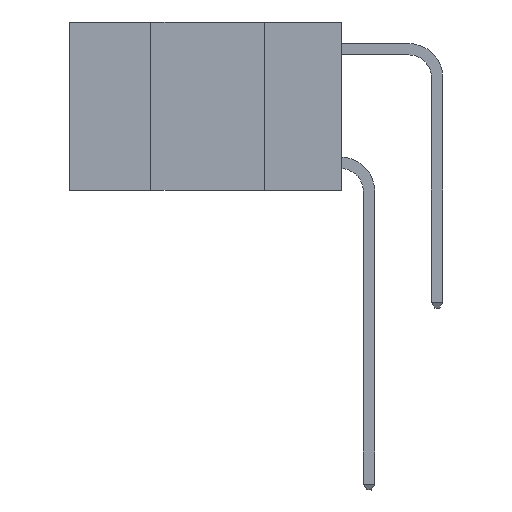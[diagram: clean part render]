
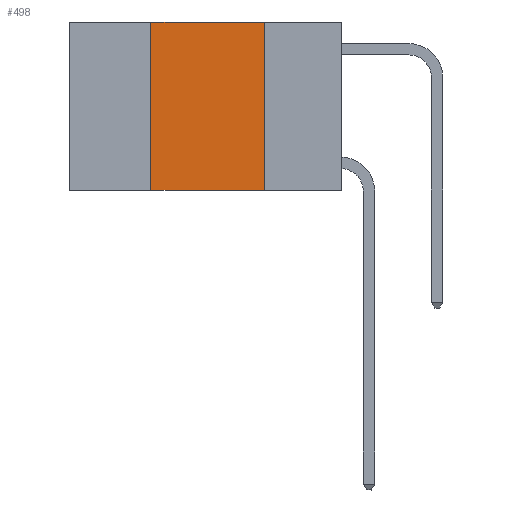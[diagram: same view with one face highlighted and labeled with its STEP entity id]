
A CAD part, left-side view. The second image highlights one B-rep face of the part: STEP entity #498.
In plain terms, the highlighted planar face has unit normal (-1, 0, 0).
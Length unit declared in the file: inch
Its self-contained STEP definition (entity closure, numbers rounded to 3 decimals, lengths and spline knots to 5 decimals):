
#15 = FACE_OUTER_BOUND ( 'NONE', #18554, .T. ) ;
#402 = DIRECTION ( 'NONE',  ( 0., -1., 0. ) ) ;
#498 = ADVANCED_FACE ( 'NONE', ( #15 ), #17483, .F. ) ;
#535 = DIRECTION ( 'NONE',  ( 0., 0., -1. ) ) ;
#1067 = VERTEX_POINT ( 'NONE', #10065 ) ;
#1711 = CARTESIAN_POINT ( 'NONE',  ( 0., 0.17, -0.37 ) ) ;
#2541 = VERTEX_POINT ( 'NONE', #13955 ) ;
#2792 = VERTEX_POINT ( 'NONE', #15150 ) ;
#3217 = LINE ( 'NONE', #16419, #7668 ) ;
#3289 = LINE ( 'NONE', #13831, #11334 ) ;
#4571 = ORIENTED_EDGE ( 'NONE', *, *, #11097, .F. ) ;
#4758 = DIRECTION ( 'NONE',  ( 0., -1., 0. ) ) ;
#4841 = DIRECTION ( 'NONE',  ( 0., 0., -1. ) ) ;
#6786 = VERTEX_POINT ( 'NONE', #1711 ) ;
#7668 = VECTOR ( 'NONE', #11910, 39.37008 ) ;
#7871 = AXIS2_PLACEMENT_3D ( 'NONE', #16072, #11118, #535 ) ;
#8346 = VECTOR ( 'NONE', #4758, 39.37008 ) ;
#8551 = EDGE_CURVE ( 'NONE', #1067, #2792, #17524, .T. ) ;
#9556 = EDGE_CURVE ( 'NONE', #2541, #1067, #3217, .T. ) ;
#10045 = ORIENTED_EDGE ( 'NONE', *, *, #9556, .F. ) ;
#10065 = CARTESIAN_POINT ( 'NONE',  ( 0., 0.42, 0. ) ) ;
#11017 = CARTESIAN_POINT ( 'NONE',  ( 0., 0.6, 0. ) ) ;
#11097 = EDGE_CURVE ( 'NONE', #2792, #6786, #3289, .T. ) ;
#11118 = DIRECTION ( 'NONE',  ( 1., 0., 0. ) ) ;
#11334 = VECTOR ( 'NONE', #4841, 39.37008 ) ;
#11910 = DIRECTION ( 'NONE',  ( 0., 0., 1. ) ) ;
#13750 = ORIENTED_EDGE ( 'NONE', *, *, #15480, .T. ) ;
#13831 = CARTESIAN_POINT ( 'NONE',  ( 0., 0.17, 0. ) ) ;
#13955 = CARTESIAN_POINT ( 'NONE',  ( 0., 0.42, -0.37 ) ) ;
#15150 = CARTESIAN_POINT ( 'NONE',  ( 0., 0.17, 0. ) ) ;
#15480 = EDGE_CURVE ( 'NONE', #2541, #6786, #16305, .T. ) ;
#16072 = CARTESIAN_POINT ( 'NONE',  ( 0., 0.6, 0. ) ) ;
#16305 = LINE ( 'NONE', #18209, #8346 ) ;
#16419 = CARTESIAN_POINT ( 'NONE',  ( 0., 0.42, 0. ) ) ;
#17064 = VECTOR ( 'NONE', #402, 39.37008 ) ;
#17483 = PLANE ( 'NONE',  #7871 ) ;
#17524 = LINE ( 'NONE', #11017, #17064 ) ;
#17564 = ORIENTED_EDGE ( 'NONE', *, *, #8551, .F. ) ;
#18209 = CARTESIAN_POINT ( 'NONE',  ( 0., 0.6, -0.37 ) ) ;
#18554 = EDGE_LOOP ( 'NONE', ( #4571, #17564, #10045, #13750 ) ) ;
